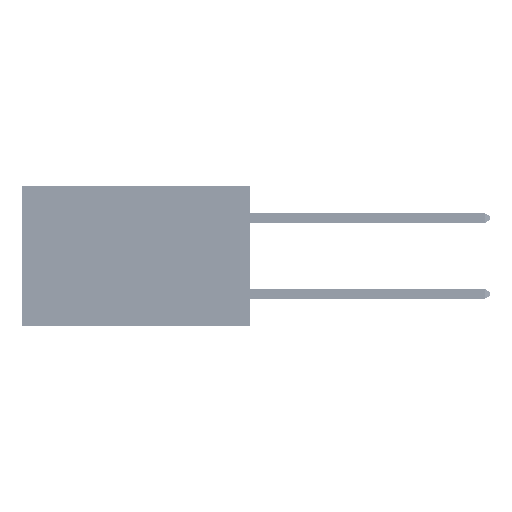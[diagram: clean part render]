
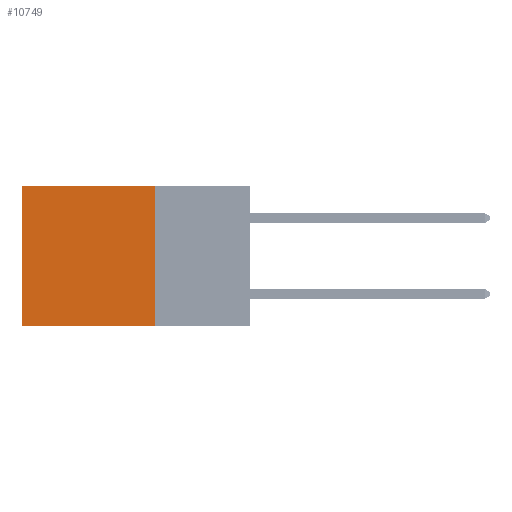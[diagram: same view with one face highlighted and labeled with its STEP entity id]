
A CAD part, left-side view. The second image highlights one B-rep face of the part: STEP entity #10749.
In plain terms, the highlighted planar face has unit normal (-1, 0, 0).
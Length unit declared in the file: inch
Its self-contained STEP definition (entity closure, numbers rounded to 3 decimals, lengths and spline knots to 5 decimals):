
#666 = ORIENTED_EDGE ( 'NONE', *, *, #37503, .F. ) ;
#705 = PLANE ( 'NONE',  #30477 ) ;
#997 = CARTESIAN_POINT ( 'NONE',  ( 0.2875, 0.25, -0.37 ) ) ;
#4156 = DIRECTION ( 'NONE',  ( 0., 0., -1. ) ) ;
#5661 = EDGE_LOOP ( 'NONE', ( #35085, #18041, #666, #15281 ) ) ;
#6947 = VERTEX_POINT ( 'NONE', #18358 ) ;
#9162 = CARTESIAN_POINT ( 'NONE',  ( 0.2875, 0.25, 0. ) ) ;
#10627 = DIRECTION ( 'NONE',  ( 0., 0., -1. ) ) ;
#10749 = ADVANCED_FACE ( 'NONE', ( #49874 ), #705, .F. ) ;
#11489 = VECTOR ( 'NONE', #20624, 39.37008 ) ;
#11694 = CARTESIAN_POINT ( 'NONE',  ( 0.2875, 0.25, 0. ) ) ;
#15109 = LINE ( 'NONE', #40654, #24357 ) ;
#15281 = ORIENTED_EDGE ( 'NONE', *, *, #42540, .T. ) ;
#18041 = ORIENTED_EDGE ( 'NONE', *, *, #22799, .F. ) ;
#18358 = CARTESIAN_POINT ( 'NONE',  ( 0.2875, 0.25, -0.37 ) ) ;
#19655 = VERTEX_POINT ( 'NONE', #45451 ) ;
#20624 = DIRECTION ( 'NONE',  ( 0., 1., 0. ) ) ;
#20747 = LINE ( 'NONE', #997, #11489 ) ;
#22072 = LINE ( 'NONE', #29958, #27606 ) ;
#22799 = EDGE_CURVE ( 'NONE', #6947, #28329, #20747, .T. ) ;
#23611 = DIRECTION ( 'NONE',  ( 0., 1., 0. ) ) ;
#24357 = VECTOR ( 'NONE', #24927, 39.37008 ) ;
#24927 = DIRECTION ( 'NONE',  ( 0., 0., -1. ) ) ;
#27606 = VECTOR ( 'NONE', #10627, 39.37008 ) ;
#28264 = DIRECTION ( 'NONE',  ( 1., 0., 0. ) ) ;
#28329 = VERTEX_POINT ( 'NONE', #48560 ) ;
#29958 = CARTESIAN_POINT ( 'NONE',  ( 0.2875, 0.25, 0. ) ) ;
#30477 = AXIS2_PLACEMENT_3D ( 'NONE', #31738, #28264, #4156 ) ;
#31349 = VERTEX_POINT ( 'NONE', #9162 ) ;
#31738 = CARTESIAN_POINT ( 'NONE',  ( 0.2875, 0.25, 0. ) ) ;
#35085 = ORIENTED_EDGE ( 'NONE', *, *, #42654, .T. ) ;
#37503 = EDGE_CURVE ( 'NONE', #31349, #6947, #22072, .T. ) ;
#40654 = CARTESIAN_POINT ( 'NONE',  ( 0.2875, 0.6, 0. ) ) ;
#42540 = EDGE_CURVE ( 'NONE', #31349, #19655, #47877, .T. ) ;
#42654 = EDGE_CURVE ( 'NONE', #19655, #28329, #15109, .T. ) ;
#45400 = VECTOR ( 'NONE', #23611, 39.37008 ) ;
#45451 = CARTESIAN_POINT ( 'NONE',  ( 0.2875, 0.6, 0. ) ) ;
#47877 = LINE ( 'NONE', #11694, #45400 ) ;
#48560 = CARTESIAN_POINT ( 'NONE',  ( 0.2875, 0.6, -0.37 ) ) ;
#49874 = FACE_OUTER_BOUND ( 'NONE', #5661, .T. ) ;
